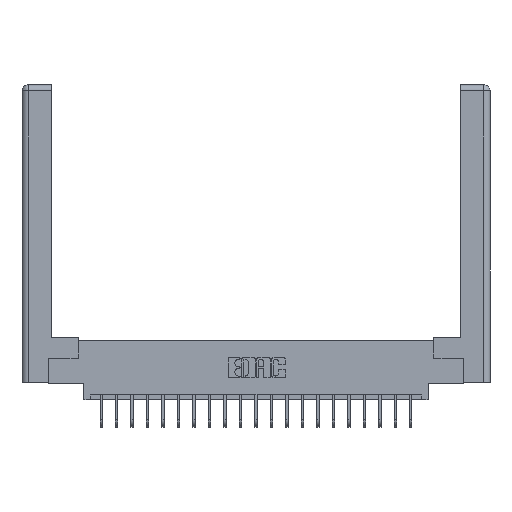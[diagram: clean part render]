
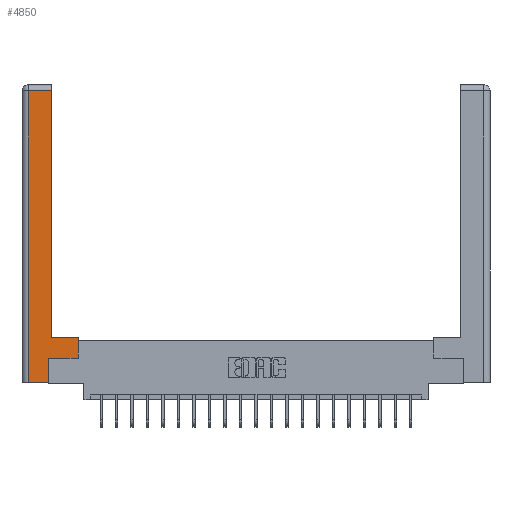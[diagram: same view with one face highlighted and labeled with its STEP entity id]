
A CAD part, top view. The second image highlights one B-rep face of the part: STEP entity #4850.
In plain terms, the highlighted planar face has unit normal (0, 0, 1).
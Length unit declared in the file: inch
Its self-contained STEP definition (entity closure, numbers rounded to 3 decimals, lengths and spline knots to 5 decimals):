
#229 = CARTESIAN_POINT ( 'NONE',  ( 0.265, 0., 0. ) ) ;
#684 = VERTEX_POINT ( 'NONE', #14949 ) ;
#719 = VECTOR ( 'NONE', #21171, 39.37008 ) ;
#841 = ORIENTED_EDGE ( 'NONE', *, *, #16641, .T. ) ;
#1294 = VERTEX_POINT ( 'NONE', #4921 ) ;
#1532 = CARTESIAN_POINT ( 'NONE',  ( 0.295, 3., 0. ) ) ;
#1980 = CARTESIAN_POINT ( 'NONE',  ( 0.295, 2.94, 0. ) ) ;
#2010 = ORIENTED_EDGE ( 'NONE', *, *, #2963, .T. ) ;
#2963 = EDGE_CURVE ( 'NONE', #7367, #20465, #15088, .T. ) ;
#3144 = CARTESIAN_POINT ( 'NONE',  ( 0.265, 0.245, 0. ) ) ;
#3767 = VERTEX_POINT ( 'NONE', #17156 ) ;
#3802 = VECTOR ( 'NONE', #15741, 39.37008 ) ;
#4356 = CARTESIAN_POINT ( 'NONE',  ( 0.265, 0., 0. ) ) ;
#4795 = EDGE_CURVE ( 'NONE', #9017, #4847, #12502, .T. ) ;
#4847 = VERTEX_POINT ( 'NONE', #9521 ) ;
#4850 = ADVANCED_FACE ( 'NONE', ( #11979 ), #17747, .F. ) ;
#4921 = CARTESIAN_POINT ( 'NONE',  ( 0.295, 0.45, 0. ) ) ;
#4963 = ORIENTED_EDGE ( 'NONE', *, *, #20054, .T. ) ;
#4985 = ORIENTED_EDGE ( 'NONE', *, *, #12372, .T. ) ;
#5397 = ORIENTED_EDGE ( 'NONE', *, *, #14588, .T. ) ;
#5643 = VECTOR ( 'NONE', #7662, 39.37008 ) ;
#6189 = LINE ( 'NONE', #229, #19749 ) ;
#6423 = VECTOR ( 'NONE', #19405, 39.37008 ) ;
#7367 = VERTEX_POINT ( 'NONE', #4356 ) ;
#7662 = DIRECTION ( 'NONE',  ( -1., 0., 0. ) ) ;
#7845 = ORIENTED_EDGE ( 'NONE', *, *, #4795, .T. ) ;
#7901 = VECTOR ( 'NONE', #12640, 39.37008 ) ;
#9017 = VERTEX_POINT ( 'NONE', #13033 ) ;
#9521 = CARTESIAN_POINT ( 'NONE',  ( 0.0615, 0., 0. ) ) ;
#9535 = DIRECTION ( 'NONE',  ( 0., -1., 0. ) ) ;
#9978 = CARTESIAN_POINT ( 'NONE',  ( 0.265, 0.245, 0. ) ) ;
#10948 = CARTESIAN_POINT ( 'NONE',  ( 0.295, 0.45, 0. ) ) ;
#11126 = CARTESIAN_POINT ( 'NONE',  ( 0.0615, 2.94, 0. ) ) ;
#11658 = DIRECTION ( 'NONE',  ( 1., 0., 0. ) ) ;
#11979 = FACE_OUTER_BOUND ( 'NONE', #20893, .T. ) ;
#12048 = LINE ( 'NONE', #11126, #5643 ) ;
#12192 = CARTESIAN_POINT ( 'NONE',  ( 0.0615, 0., 0. ) ) ;
#12372 = EDGE_CURVE ( 'NONE', #3767, #684, #13277, .T. ) ;
#12502 = LINE ( 'NONE', #12192, #13992 ) ;
#12640 = DIRECTION ( 'NONE',  ( 0., 1., 0. ) ) ;
#12902 = CARTESIAN_POINT ( 'NONE',  ( 0., 0., 0. ) ) ;
#12916 = CARTESIAN_POINT ( 'NONE',  ( 0.565, 0.245, 0. ) ) ;
#13033 = CARTESIAN_POINT ( 'NONE',  ( 0.0615, 2.94, 0. ) ) ;
#13277 = LINE ( 'NONE', #17397, #7901 ) ;
#13575 = LINE ( 'NONE', #12916, #6423 ) ;
#13992 = VECTOR ( 'NONE', #9535, 39.37008 ) ;
#14508 = ORIENTED_EDGE ( 'NONE', *, *, #17381, .T. ) ;
#14510 = DIRECTION ( 'NONE',  ( 0., 1., 0. ) ) ;
#14588 = EDGE_CURVE ( 'NONE', #20465, #3767, #13575, .T. ) ;
#14779 = VERTEX_POINT ( 'NONE', #1980 ) ;
#14949 = CARTESIAN_POINT ( 'NONE',  ( 0.565, 0.45, 0. ) ) ;
#15088 = LINE ( 'NONE', #3144, #18952 ) ;
#15103 = EDGE_CURVE ( 'NONE', #14779, #9017, #12048, .T. ) ;
#15245 = LINE ( 'NONE', #10948, #3802 ) ;
#15741 = DIRECTION ( 'NONE',  ( -1., 0., 0. ) ) ;
#16641 = EDGE_CURVE ( 'NONE', #684, #1294, #15245, .T. ) ;
#17025 = LINE ( 'NONE', #1532, #719 ) ;
#17156 = CARTESIAN_POINT ( 'NONE',  ( 0.565, 0.245, 0. ) ) ;
#17381 = EDGE_CURVE ( 'NONE', #1294, #14779, #17025, .T. ) ;
#17397 = CARTESIAN_POINT ( 'NONE',  ( 0.565, 0.45, 0. ) ) ;
#17747 = PLANE ( 'NONE',  #18752 ) ;
#18752 = AXIS2_PLACEMENT_3D ( 'NONE', #12902, #19388, #21047 ) ;
#18952 = VECTOR ( 'NONE', #14510, 39.37008 ) ;
#19388 = DIRECTION ( 'NONE',  ( 0., 0., -1. ) ) ;
#19405 = DIRECTION ( 'NONE',  ( 1., 0., 0. ) ) ;
#19749 = VECTOR ( 'NONE', #11658, 39.37008 ) ;
#20054 = EDGE_CURVE ( 'NONE', #4847, #7367, #6189, .T. ) ;
#20465 = VERTEX_POINT ( 'NONE', #9978 ) ;
#20716 = ORIENTED_EDGE ( 'NONE', *, *, #15103, .T. ) ;
#20893 = EDGE_LOOP ( 'NONE', ( #14508, #20716, #7845, #4963, #2010, #5397, #4985, #841 ) ) ;
#21047 = DIRECTION ( 'NONE',  ( -1., 0., 0. ) ) ;
#21171 = DIRECTION ( 'NONE',  ( 0., 1., 0. ) ) ;
